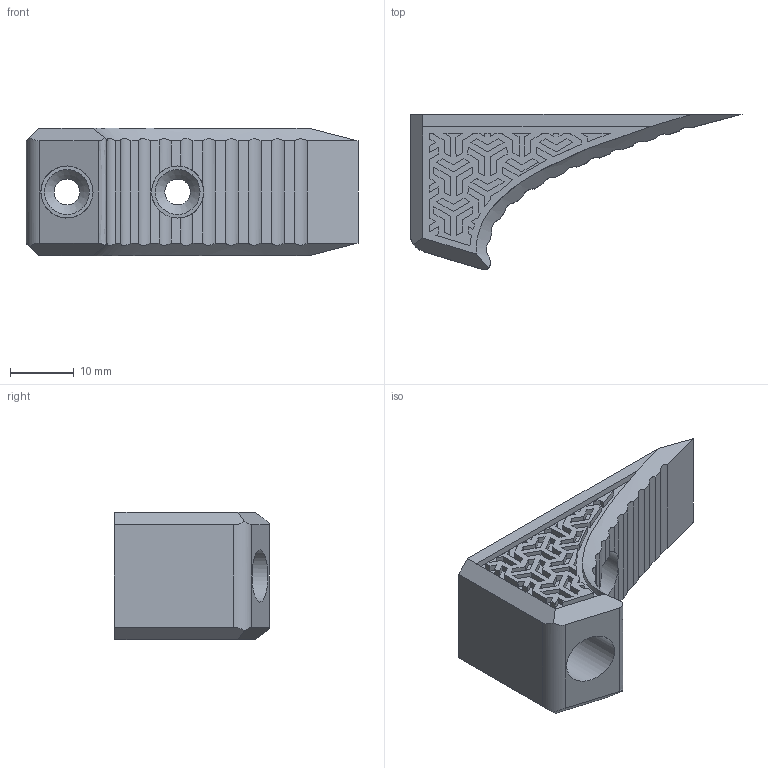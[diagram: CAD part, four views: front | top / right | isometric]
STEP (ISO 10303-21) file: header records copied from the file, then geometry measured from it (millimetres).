
FILE_DESCRIPTION(/* description */ (''),/* implementation_level */ '2;1');
FILE_NAME(/* name */ 'Small Hand Stop.step',/* time_stamp */ '2022-05-12T11:10:00-06:00',/* author */ (''),/* organization */ (''),/* preprocessor_version */ 'ST-DEVELOPER v18.1',/* originating_system */ 'Autodesk Translation Framework v10.10.0.1391',/* authorisation */ '');
FILE_SCHEMA (('AUTOMOTIVE_DESIGN { 1 0 10303 214 3 1 1 }'));
Length unit declared in the file: millimetre
Products named in the file (1): Hand stop
Bounding box: 51.93 x 24.33 x 20 mm (x, y, z)
Volume: 8757.3 mm3; surface area: 5028.4 mm2
Topology: 1 solids, 1 shells, 432 faces, 1194 edges, 793 vertices
Faces by surface type: plane 377, bspline 35, cylinder 18, cone 2
Full cylindrical faces by diameter (mm): 4 x2, 8.15 x2
Entity records: 15391 total; most frequent: CARTESIAN_POINT 4681, ORIENTED_EDGE 2388, DIRECTION 1864, EDGE_CURVE 1194, LINE 1042, VECTOR 1042, VERTEX_POINT 793, EDGE_LOOP 465
